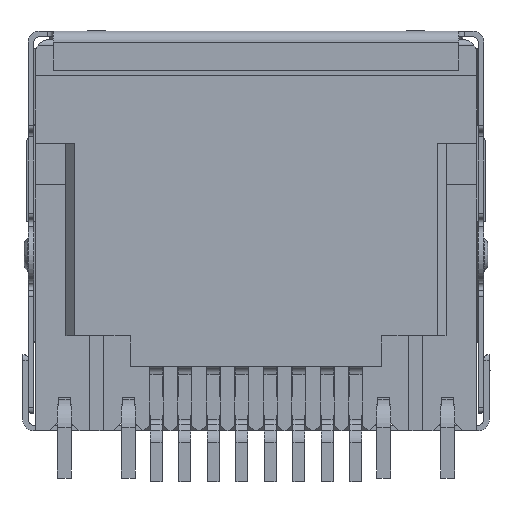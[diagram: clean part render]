
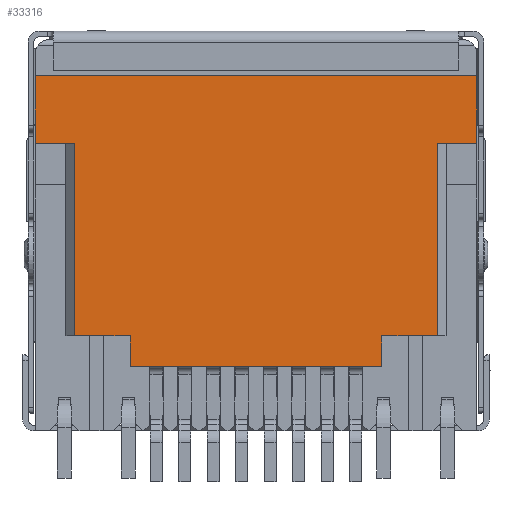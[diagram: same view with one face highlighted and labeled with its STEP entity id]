
A CAD part, front view. The second image highlights one B-rep face of the part: STEP entity #33316.
In plain terms, the highlighted planar face has unit normal (0, -1, 0).
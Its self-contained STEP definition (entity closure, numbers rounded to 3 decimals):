
#1255 = LINE ( 'NONE', #11312, #29820 ) ;
#1823 = VERTEX_POINT ( 'NONE', #18015 ) ;
#2517 = LINE ( 'NONE', #37594, #30511 ) ;
#2574 = EDGE_LOOP ( 'NONE', ( #42661, #39094, #10456, #8525, #40110, #36392, #18984, #17933, #25476, #9566, #4250, #49731 ) ) ;
#2949 = DIRECTION ( 'NONE',  ( 0., 0., -1. ) ) ;
#2989 = EDGE_CURVE ( 'NONE', #14609, #44603, #45657, .T. ) ;
#3084 = VECTOR ( 'NONE', #4688, 1000. ) ;
#3293 = VECTOR ( 'NONE', #49837, 1000. ) ;
#3730 = EDGE_CURVE ( 'NONE', #1823, #9835, #20938, .T. ) ;
#3756 = DIRECTION ( 'NONE',  ( 1., 0., 0. ) ) ;
#4250 = ORIENTED_EDGE ( 'NONE', *, *, #24829, .T. ) ;
#4688 = DIRECTION ( 'NONE',  ( 0., 0., 1. ) ) ;
#5057 = DIRECTION ( 'NONE',  ( 1., 0., 0. ) ) ;
#5242 = CARTESIAN_POINT ( 'NONE',  ( 7.9, -5.525, -3.7 ) ) ;
#5317 = EDGE_CURVE ( 'NONE', #45356, #50125, #2517, .T. ) ;
#6436 = VECTOR ( 'NONE', #16813, 1000. ) ;
#7255 = EDGE_CURVE ( 'NONE', #50125, #40887, #1255, .T. ) ;
#8525 = ORIENTED_EDGE ( 'NONE', *, *, #47855, .F. ) ;
#9566 = ORIENTED_EDGE ( 'NONE', *, *, #25121, .T. ) ;
#9835 = VERTEX_POINT ( 'NONE', #47259 ) ;
#10094 = CARTESIAN_POINT ( 'NONE',  ( -7.9, -5.525, -1.3 ) ) ;
#10456 = ORIENTED_EDGE ( 'NONE', *, *, #3730, .T. ) ;
#11186 = CARTESIAN_POINT ( 'NONE',  ( 4.5, -5.525, -10.6 ) ) ;
#11312 = CARTESIAN_POINT ( 'NONE',  ( -6.5, -5.525, -14. ) ) ;
#11432 = LINE ( 'NONE', #22263, #26022 ) ;
#11642 = EDGE_CURVE ( 'NONE', #40887, #43658, #42037, .T. ) ;
#11915 = CARTESIAN_POINT ( 'NONE',  ( -4.5, -5.525, -10.6 ) ) ;
#13058 = VERTEX_POINT ( 'NONE', #37134 ) ;
#14423 = VERTEX_POINT ( 'NONE', #27170 ) ;
#14609 = VERTEX_POINT ( 'NONE', #31549 ) ;
#14817 = PLANE ( 'NONE',  #38732 ) ;
#15460 = VECTOR ( 'NONE', #40357, 1000. ) ;
#16654 = CARTESIAN_POINT ( 'NONE',  ( -7.9, -5.525, -10.6 ) ) ;
#16791 = LINE ( 'NONE', #16654, #6436 ) ;
#16813 = DIRECTION ( 'NONE',  ( 1., 0., 0. ) ) ;
#17474 = CARTESIAN_POINT ( 'NONE',  ( -7.9, -5.525, -11.7 ) ) ;
#17665 = EDGE_CURVE ( 'NONE', #43967, #14423, #42212, .T. ) ;
#17762 = CARTESIAN_POINT ( 'NONE',  ( 6.5, -5.525, -3.7 ) ) ;
#17933 = ORIENTED_EDGE ( 'NONE', *, *, #36649, .T. ) ;
#17937 = VECTOR ( 'NONE', #49236, 1000. ) ;
#18015 = CARTESIAN_POINT ( 'NONE',  ( 7.9, -5.525, -1.3 ) ) ;
#18375 = DIRECTION ( 'NONE',  ( 0., 0., 1. ) ) ;
#18920 = CARTESIAN_POINT ( 'NONE',  ( -7.9, -5.525, -14. ) ) ;
#18984 = ORIENTED_EDGE ( 'NONE', *, *, #11642, .T. ) ;
#20938 = LINE ( 'NONE', #10094, #15460 ) ;
#22263 = CARTESIAN_POINT ( 'NONE',  ( -7.9, -5.525, -3.7 ) ) ;
#22361 = CARTESIAN_POINT ( 'NONE',  ( 7.9, -5.525, -14. ) ) ;
#22830 = DIRECTION ( 'NONE',  ( 0., -1., 0. ) ) ;
#22855 = CARTESIAN_POINT ( 'NONE',  ( -6.5, -5.525, -3.7 ) ) ;
#23363 = FACE_OUTER_BOUND ( 'NONE', #2574, .T. ) ;
#24829 = EDGE_CURVE ( 'NONE', #13058, #14609, #16791, .T. ) ;
#25121 = EDGE_CURVE ( 'NONE', #14423, #13058, #42315, .T. ) ;
#25476 = ORIENTED_EDGE ( 'NONE', *, *, #17665, .T. ) ;
#26022 = VECTOR ( 'NONE', #26192, 1000. ) ;
#26192 = DIRECTION ( 'NONE',  ( 1., 0., 0. ) ) ;
#27113 = LINE ( 'NONE', #22361, #17937 ) ;
#27170 = CARTESIAN_POINT ( 'NONE',  ( 4.5, -5.525, -11.7 ) ) ;
#27461 = VERTEX_POINT ( 'NONE', #5242 ) ;
#27508 = CARTESIAN_POINT ( 'NONE',  ( -7.9, -5.525, -14. ) ) ;
#29820 = VECTOR ( 'NONE', #50089, 1000. ) ;
#30428 = VECTOR ( 'NONE', #18375, 1000. ) ;
#30511 = VECTOR ( 'NONE', #3756, 1000. ) ;
#31549 = CARTESIAN_POINT ( 'NONE',  ( 6.5, -5.525, -10.6 ) ) ;
#33316 = ADVANCED_FACE ( 'NONE', ( #23363 ), #14817, .T. ) ;
#36392 = ORIENTED_EDGE ( 'NONE', *, *, #7255, .T. ) ;
#36649 = EDGE_CURVE ( 'NONE', #43658, #43967, #39511, .T. ) ;
#37134 = CARTESIAN_POINT ( 'NONE',  ( 4.5, -5.525, -10.6 ) ) ;
#37594 = CARTESIAN_POINT ( 'NONE',  ( -7.9, -5.525, -3.7 ) ) ;
#38732 = AXIS2_PLACEMENT_3D ( 'NONE', #18920, #22830, #2949 ) ;
#39094 = ORIENTED_EDGE ( 'NONE', *, *, #43220, .F. ) ;
#39511 = LINE ( 'NONE', #11915, #48013 ) ;
#39587 = CARTESIAN_POINT ( 'NONE',  ( -7.9, -5.525, -10.6 ) ) ;
#39814 = CARTESIAN_POINT ( 'NONE',  ( -4.5, -5.525, -11.7 ) ) ;
#40110 = ORIENTED_EDGE ( 'NONE', *, *, #5317, .T. ) ;
#40357 = DIRECTION ( 'NONE',  ( -1., 0., 0. ) ) ;
#40887 = VERTEX_POINT ( 'NONE', #45871 ) ;
#41676 = CARTESIAN_POINT ( 'NONE',  ( 6.5, -5.525, -14. ) ) ;
#41809 = EDGE_CURVE ( 'NONE', #44603, #27461, #11432, .T. ) ;
#42037 = LINE ( 'NONE', #39587, #48153 ) ;
#42212 = LINE ( 'NONE', #17474, #3293 ) ;
#42292 = DIRECTION ( 'NONE',  ( 0., 0., 1. ) ) ;
#42315 = LINE ( 'NONE', #11186, #42952 ) ;
#42661 = ORIENTED_EDGE ( 'NONE', *, *, #41809, .T. ) ;
#42952 = VECTOR ( 'NONE', #42292, 1000. ) ;
#43220 = EDGE_CURVE ( 'NONE', #1823, #27461, #27113, .T. ) ;
#43658 = VERTEX_POINT ( 'NONE', #49509 ) ;
#43967 = VERTEX_POINT ( 'NONE', #39814 ) ;
#44603 = VERTEX_POINT ( 'NONE', #17762 ) ;
#45356 = VERTEX_POINT ( 'NONE', #50386 ) ;
#45594 = DIRECTION ( 'NONE',  ( 0., 0., -1. ) ) ;
#45657 = LINE ( 'NONE', #41676, #30428 ) ;
#45871 = CARTESIAN_POINT ( 'NONE',  ( -6.5, -5.525, -10.6 ) ) ;
#46905 = LINE ( 'NONE', #27508, #3084 ) ;
#47259 = CARTESIAN_POINT ( 'NONE',  ( -7.9, -5.525, -1.3 ) ) ;
#47855 = EDGE_CURVE ( 'NONE', #45356, #9835, #46905, .T. ) ;
#48013 = VECTOR ( 'NONE', #45594, 1000. ) ;
#48153 = VECTOR ( 'NONE', #5057, 1000. ) ;
#49236 = DIRECTION ( 'NONE',  ( 0., 0., -1. ) ) ;
#49509 = CARTESIAN_POINT ( 'NONE',  ( -4.5, -5.525, -10.6 ) ) ;
#49731 = ORIENTED_EDGE ( 'NONE', *, *, #2989, .T. ) ;
#49837 = DIRECTION ( 'NONE',  ( 1., 0., 0. ) ) ;
#50089 = DIRECTION ( 'NONE',  ( 0., 0., -1. ) ) ;
#50125 = VERTEX_POINT ( 'NONE', #22855 ) ;
#50386 = CARTESIAN_POINT ( 'NONE',  ( -7.9, -5.525, -3.7 ) ) ;
